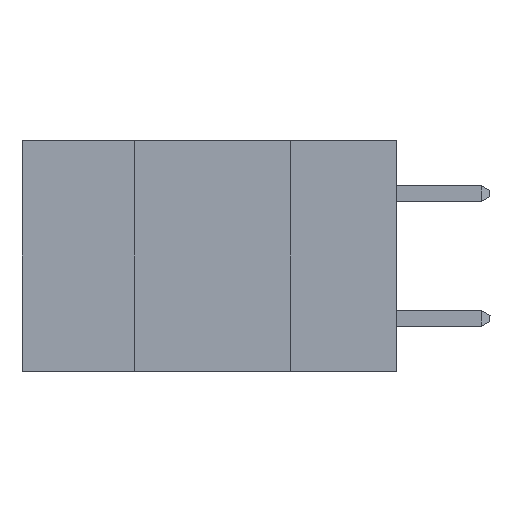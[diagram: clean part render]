
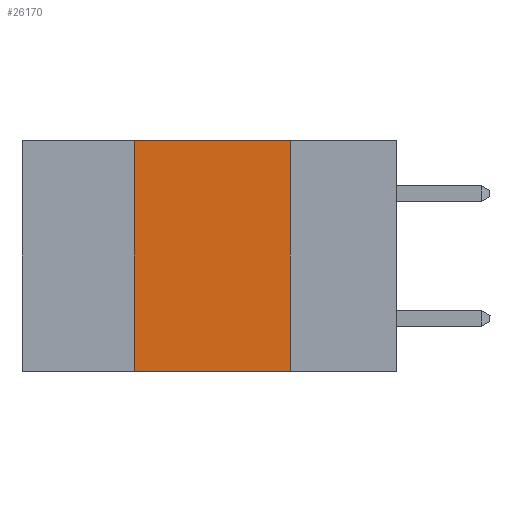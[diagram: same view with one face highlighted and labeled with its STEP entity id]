
A CAD part, left-side view. The second image highlights one B-rep face of the part: STEP entity #26170.
In plain terms, the highlighted planar face has unit normal (-1, 0, 0).
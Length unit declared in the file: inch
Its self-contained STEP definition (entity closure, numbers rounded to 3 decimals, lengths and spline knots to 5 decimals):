
#415 = CARTESIAN_POINT ( 'NONE',  ( 0., 0.42, 0. ) ) ;
#1516 = VECTOR ( 'NONE', #20748, 39.37008 ) ;
#1523 = CARTESIAN_POINT ( 'NONE',  ( 0., 0.42, -0.37 ) ) ;
#2584 = DIRECTION ( 'NONE',  ( 0., 0., 1. ) ) ;
#3040 = VERTEX_POINT ( 'NONE', #7607 ) ;
#3404 = CARTESIAN_POINT ( 'NONE',  ( 0., 0.42, 0. ) ) ;
#3630 = EDGE_LOOP ( 'NONE', ( #11105, #16816, #21183, #13224 ) ) ;
#4605 = LINE ( 'NONE', #10663, #6199 ) ;
#6199 = VECTOR ( 'NONE', #6726, 39.37008 ) ;
#6323 = EDGE_CURVE ( 'NONE', #24816, #17503, #24191, .T. ) ;
#6726 = DIRECTION ( 'NONE',  ( 0., -1., 0. ) ) ;
#7081 = VECTOR ( 'NONE', #12863, 39.37008 ) ;
#7607 = CARTESIAN_POINT ( 'NONE',  ( 0., 0.17, -0.37 ) ) ;
#7876 = LINE ( 'NONE', #12966, #1516 ) ;
#10663 = CARTESIAN_POINT ( 'NONE',  ( 0., 0.6, -0.37 ) ) ;
#10882 = AXIS2_PLACEMENT_3D ( 'NONE', #18634, #12256, #14315 ) ;
#11105 = ORIENTED_EDGE ( 'NONE', *, *, #11796, .F. ) ;
#11796 = EDGE_CURVE ( 'NONE', #17503, #3040, #7876, .T. ) ;
#12256 = DIRECTION ( 'NONE',  ( 1., 0., 0. ) ) ;
#12863 = DIRECTION ( 'NONE',  ( 0., -1., 0. ) ) ;
#12966 = CARTESIAN_POINT ( 'NONE',  ( 0., 0.17, 0. ) ) ;
#13224 = ORIENTED_EDGE ( 'NONE', *, *, #18328, .T. ) ;
#14315 = DIRECTION ( 'NONE',  ( 0., 0., -1. ) ) ;
#15148 = VECTOR ( 'NONE', #2584, 39.37008 ) ;
#15182 = VERTEX_POINT ( 'NONE', #1523 ) ;
#16816 = ORIENTED_EDGE ( 'NONE', *, *, #6323, .F. ) ;
#17503 = VERTEX_POINT ( 'NONE', #24783 ) ;
#18328 = EDGE_CURVE ( 'NONE', #15182, #3040, #4605, .T. ) ;
#18634 = CARTESIAN_POINT ( 'NONE',  ( 0., 0.6, 0. ) ) ;
#20529 = LINE ( 'NONE', #415, #15148 ) ;
#20748 = DIRECTION ( 'NONE',  ( 0., 0., -1. ) ) ;
#21183 = ORIENTED_EDGE ( 'NONE', *, *, #25040, .F. ) ;
#22362 = FACE_OUTER_BOUND ( 'NONE', #3630, .T. ) ;
#22737 = CARTESIAN_POINT ( 'NONE',  ( 0., 0.6, 0. ) ) ;
#24191 = LINE ( 'NONE', #22737, #7081 ) ;
#24710 = PLANE ( 'NONE',  #10882 ) ;
#24783 = CARTESIAN_POINT ( 'NONE',  ( 0., 0.17, 0. ) ) ;
#24816 = VERTEX_POINT ( 'NONE', #3404 ) ;
#25040 = EDGE_CURVE ( 'NONE', #15182, #24816, #20529, .T. ) ;
#26170 = ADVANCED_FACE ( 'NONE', ( #22362 ), #24710, .F. ) ;
